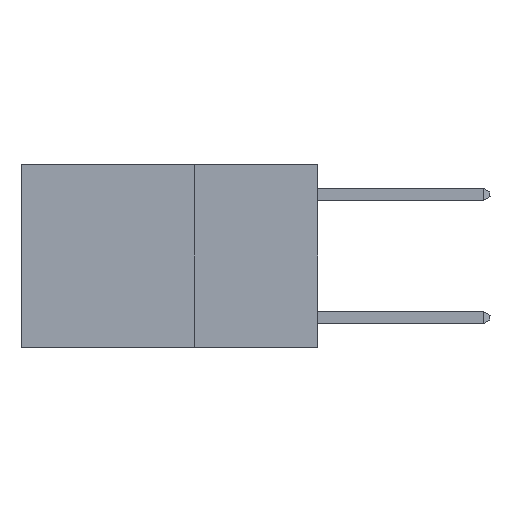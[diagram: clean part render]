
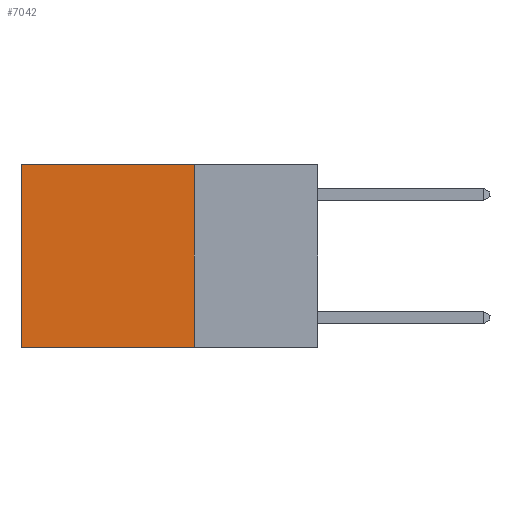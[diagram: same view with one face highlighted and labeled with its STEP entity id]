
A CAD part, left-side view. The second image highlights one B-rep face of the part: STEP entity #7042.
In plain terms, the highlighted planar face has unit normal (-1, 0, 0).
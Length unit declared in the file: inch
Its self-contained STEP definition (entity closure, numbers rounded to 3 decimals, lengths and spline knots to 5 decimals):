
#899 = CARTESIAN_POINT ( 'NONE',  ( 0.2625, 0.25, 0. ) ) ;
#902 = DIRECTION ( 'NONE',  ( 0., 0., -1. ) ) ;
#941 = CARTESIAN_POINT ( 'NONE',  ( 0.2625, 0.25, -0.37 ) ) ;
#1003 = DIRECTION ( 'NONE',  ( 0., 0., -1. ) ) ;
#1447 = LINE ( 'NONE', #4688, #16799 ) ;
#2356 = EDGE_CURVE ( 'NONE', #12636, #19599, #12842, .T. ) ;
#2584 = LINE ( 'NONE', #4596, #17679 ) ;
#4596 = CARTESIAN_POINT ( 'NONE',  ( 0.2625, 0.25, 0. ) ) ;
#4688 = CARTESIAN_POINT ( 'NONE',  ( 0.2625, 0.6, 0. ) ) ;
#4783 = ORIENTED_EDGE ( 'NONE', *, *, #15868, .T. ) ;
#5338 = ORIENTED_EDGE ( 'NONE', *, *, #14640, .F. ) ;
#7042 = ADVANCED_FACE ( 'NONE', ( #15033 ), #21890, .F. ) ;
#7365 = DIRECTION ( 'NONE',  ( 0., 1., 0. ) ) ;
#10273 = VERTEX_POINT ( 'NONE', #15630 ) ;
#11003 = VECTOR ( 'NONE', #18670, 39.37008 ) ;
#11846 = LINE ( 'NONE', #19105, #11003 ) ;
#12292 = EDGE_CURVE ( 'NONE', #10273, #19599, #1447, .T. ) ;
#12612 = VERTEX_POINT ( 'NONE', #17485 ) ;
#12627 = ORIENTED_EDGE ( 'NONE', *, *, #2356, .F. ) ;
#12636 = VERTEX_POINT ( 'NONE', #15902 ) ;
#12813 = DIRECTION ( 'NONE',  ( 1., 0., 0. ) ) ;
#12842 = LINE ( 'NONE', #941, #17372 ) ;
#14467 = AXIS2_PLACEMENT_3D ( 'NONE', #899, #12813, #19865 ) ;
#14640 = EDGE_CURVE ( 'NONE', #12612, #12636, #2584, .T. ) ;
#15033 = FACE_OUTER_BOUND ( 'NONE', #19507, .T. ) ;
#15630 = CARTESIAN_POINT ( 'NONE',  ( 0.2625, 0.6, 0. ) ) ;
#15868 = EDGE_CURVE ( 'NONE', #12612, #10273, #11846, .T. ) ;
#15902 = CARTESIAN_POINT ( 'NONE',  ( 0.2625, 0.25, -0.37 ) ) ;
#16799 = VECTOR ( 'NONE', #1003, 39.37008 ) ;
#17372 = VECTOR ( 'NONE', #7365, 39.37008 ) ;
#17485 = CARTESIAN_POINT ( 'NONE',  ( 0.2625, 0.25, 0. ) ) ;
#17679 = VECTOR ( 'NONE', #902, 39.37008 ) ;
#18670 = DIRECTION ( 'NONE',  ( 0., 1., 0. ) ) ;
#19105 = CARTESIAN_POINT ( 'NONE',  ( 0.2625, 0.25, 0. ) ) ;
#19507 = EDGE_LOOP ( 'NONE', ( #21188, #12627, #5338, #4783 ) ) ;
#19599 = VERTEX_POINT ( 'NONE', #20828 ) ;
#19865 = DIRECTION ( 'NONE',  ( 0., 0., -1. ) ) ;
#20828 = CARTESIAN_POINT ( 'NONE',  ( 0.2625, 0.6, -0.37 ) ) ;
#21188 = ORIENTED_EDGE ( 'NONE', *, *, #12292, .T. ) ;
#21890 = PLANE ( 'NONE',  #14467 ) ;
